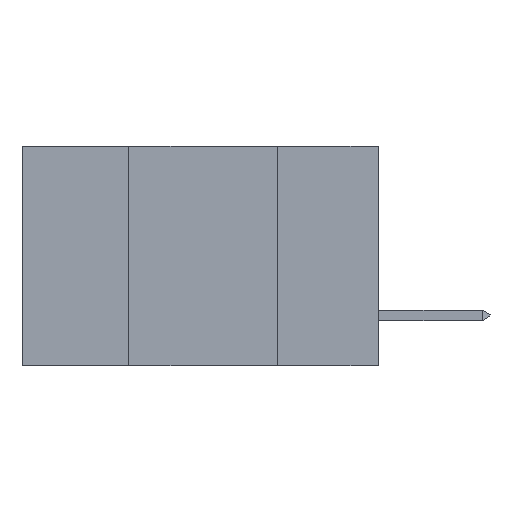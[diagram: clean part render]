
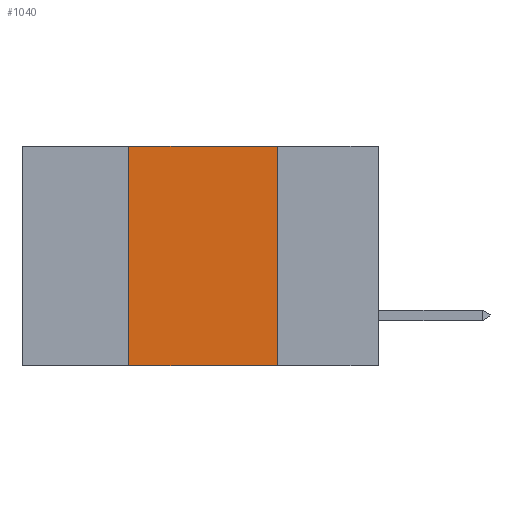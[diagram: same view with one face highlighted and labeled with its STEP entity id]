
A CAD part, left-side view. The second image highlights one B-rep face of the part: STEP entity #1040.
In plain terms, the highlighted planar face has unit normal (-1, 0, 0).
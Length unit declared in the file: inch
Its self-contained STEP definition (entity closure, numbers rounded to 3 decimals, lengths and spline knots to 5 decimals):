
#634 = PLANE ( 'NONE',  #15133 ) ;
#702 = CARTESIAN_POINT ( 'NONE',  ( 0., 0.6, 0. ) ) ;
#867 = CARTESIAN_POINT ( 'NONE',  ( 0., 0.42, 0. ) ) ;
#885 = DIRECTION ( 'NONE',  ( 0., -1., 0. ) ) ;
#1040 = ADVANCED_FACE ( 'NONE', ( #8949 ), #634, .F. ) ;
#1298 = VECTOR ( 'NONE', #11000, 39.37008 ) ;
#1352 = VERTEX_POINT ( 'NONE', #12985 ) ;
#1815 = EDGE_CURVE ( 'NONE', #14361, #7864, #14249, .T. ) ;
#2196 = ORIENTED_EDGE ( 'NONE', *, *, #5714, .F. ) ;
#3284 = VERTEX_POINT ( 'NONE', #11925 ) ;
#4866 = CARTESIAN_POINT ( 'NONE',  ( 0., 0.6, -0.37 ) ) ;
#5056 = LINE ( 'NONE', #11535, #8669 ) ;
#5203 = EDGE_CURVE ( 'NONE', #1352, #3284, #13439, .T. ) ;
#5714 = EDGE_CURVE ( 'NONE', #7864, #3284, #5056, .T. ) ;
#6074 = DIRECTION ( 'NONE',  ( 0., -1., 0. ) ) ;
#6132 = CARTESIAN_POINT ( 'NONE',  ( 0., 0.42, -0.37 ) ) ;
#7864 = VERTEX_POINT ( 'NONE', #15136 ) ;
#7967 = ORIENTED_EDGE ( 'NONE', *, *, #1815, .F. ) ;
#8669 = VECTOR ( 'NONE', #13952, 39.37008 ) ;
#8949 = FACE_OUTER_BOUND ( 'NONE', #11715, .T. ) ;
#9187 = DIRECTION ( 'NONE',  ( 1., 0., 0. ) ) ;
#10448 = EDGE_CURVE ( 'NONE', #1352, #14361, #13414, .T. ) ;
#11000 = DIRECTION ( 'NONE',  ( 0., 0., 1. ) ) ;
#11519 = CARTESIAN_POINT ( 'NONE',  ( 0., 0.6, 0. ) ) ;
#11535 = CARTESIAN_POINT ( 'NONE',  ( 0., 0.17, -0.37 ) ) ;
#11696 = ORIENTED_EDGE ( 'NONE', *, *, #10448, .F. ) ;
#11715 = EDGE_LOOP ( 'NONE', ( #2196, #7967, #11696, #13779 ) ) ;
#11718 = VECTOR ( 'NONE', #6074, 39.37008 ) ;
#11925 = CARTESIAN_POINT ( 'NONE',  ( 0., 0.17, -0.37 ) ) ;
#12985 = CARTESIAN_POINT ( 'NONE',  ( 0., 0.42, -0.37 ) ) ;
#13414 = LINE ( 'NONE', #6132, #1298 ) ;
#13439 = LINE ( 'NONE', #4866, #11718 ) ;
#13779 = ORIENTED_EDGE ( 'NONE', *, *, #5203, .T. ) ;
#13952 = DIRECTION ( 'NONE',  ( 0., 0., -1. ) ) ;
#13967 = VECTOR ( 'NONE', #885, 39.37008 ) ;
#14073 = DIRECTION ( 'NONE',  ( 0., 0., -1. ) ) ;
#14249 = LINE ( 'NONE', #11519, #13967 ) ;
#14361 = VERTEX_POINT ( 'NONE', #867 ) ;
#15133 = AXIS2_PLACEMENT_3D ( 'NONE', #702, #9187, #14073 ) ;
#15136 = CARTESIAN_POINT ( 'NONE',  ( 0., 0.17, 0. ) ) ;
